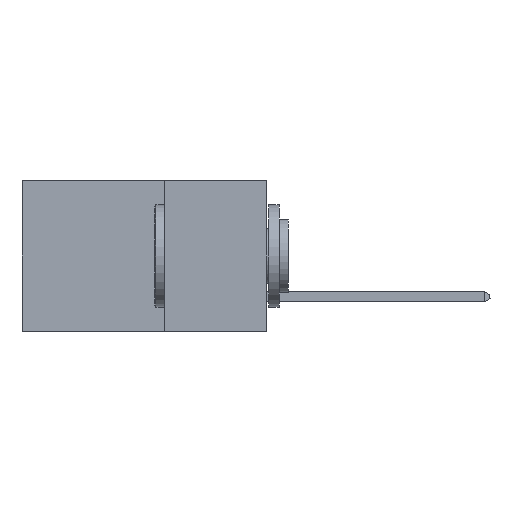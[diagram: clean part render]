
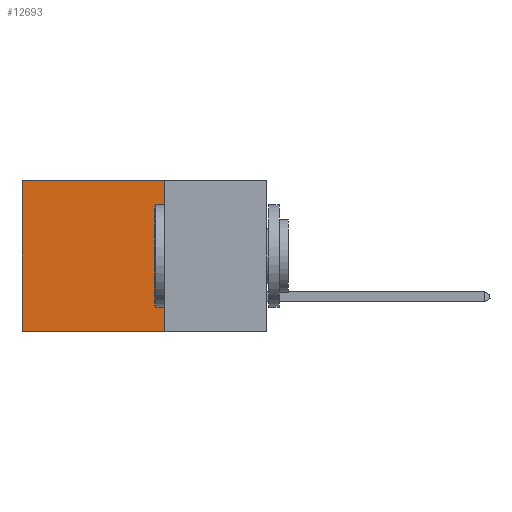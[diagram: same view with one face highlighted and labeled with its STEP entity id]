
A CAD part, left-side view. The second image highlights one B-rep face of the part: STEP entity #12693.
In plain terms, the highlighted planar face has unit normal (-1, 0, 0).
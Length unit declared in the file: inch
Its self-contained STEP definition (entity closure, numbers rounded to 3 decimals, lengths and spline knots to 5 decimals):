
#248 = LINE ( 'NONE', #10820, #5855 ) ;
#444 = CARTESIAN_POINT ( 'NONE',  ( 0.2875, 0.6, 0. ) ) ;
#707 = CARTESIAN_POINT ( 'NONE',  ( 0.2875, 0.6, -0.37 ) ) ;
#848 = ORIENTED_EDGE ( 'NONE', *, *, #1174, .T. ) ;
#1150 = EDGE_CURVE ( 'NONE', #14687, #1339, #15746, .T. ) ;
#1174 = EDGE_CURVE ( 'NONE', #4764, #14687, #248, .T. ) ;
#1325 = LINE ( 'NONE', #12075, #5479 ) ;
#1339 = VERTEX_POINT ( 'NONE', #707 ) ;
#1857 = CARTESIAN_POINT ( 'NONE',  ( 0.2875, 0.25, 0. ) ) ;
#2136 = LINE ( 'NONE', #1857, #9695 ) ;
#2764 = VERTEX_POINT ( 'NONE', #3407 ) ;
#3035 = CARTESIAN_POINT ( 'NONE',  ( 0.2875, 0.6, 0. ) ) ;
#3171 = DIRECTION ( 'NONE',  ( 0., 1., 0. ) ) ;
#3407 = CARTESIAN_POINT ( 'NONE',  ( 0.2875, 0.25, -0.37 ) ) ;
#4142 = EDGE_CURVE ( 'NONE', #4764, #2764, #2136, .T. ) ;
#4764 = VERTEX_POINT ( 'NONE', #6896 ) ;
#5479 = VECTOR ( 'NONE', #3171, 39.37008 ) ;
#5855 = VECTOR ( 'NONE', #9443, 39.37008 ) ;
#6426 = CARTESIAN_POINT ( 'NONE',  ( 0.2875, 0.25, 0. ) ) ;
#6896 = CARTESIAN_POINT ( 'NONE',  ( 0.2875, 0.25, 0. ) ) ;
#7521 = EDGE_LOOP ( 'NONE', ( #8079, #8293, #14871, #848 ) ) ;
#7677 = DIRECTION ( 'NONE',  ( 0., 0., -1. ) ) ;
#8079 = ORIENTED_EDGE ( 'NONE', *, *, #1150, .T. ) ;
#8144 = FACE_OUTER_BOUND ( 'NONE', #7521, .T. ) ;
#8293 = ORIENTED_EDGE ( 'NONE', *, *, #14139, .F. ) ;
#9443 = DIRECTION ( 'NONE',  ( 0., 1., 0. ) ) ;
#9467 = DIRECTION ( 'NONE',  ( 0., 0., -1. ) ) ;
#9695 = VECTOR ( 'NONE', #9467, 39.37008 ) ;
#10820 = CARTESIAN_POINT ( 'NONE',  ( 0.2875, 0.25, 0. ) ) ;
#11188 = AXIS2_PLACEMENT_3D ( 'NONE', #6426, #15168, #7677 ) ;
#11527 = PLANE ( 'NONE',  #11188 ) ;
#12075 = CARTESIAN_POINT ( 'NONE',  ( 0.2875, 0.25, -0.37 ) ) ;
#12596 = VECTOR ( 'NONE', #15952, 39.37008 ) ;
#12693 = ADVANCED_FACE ( 'NONE', ( #8144 ), #11527, .F. ) ;
#14139 = EDGE_CURVE ( 'NONE', #2764, #1339, #1325, .T. ) ;
#14687 = VERTEX_POINT ( 'NONE', #3035 ) ;
#14871 = ORIENTED_EDGE ( 'NONE', *, *, #4142, .F. ) ;
#15168 = DIRECTION ( 'NONE',  ( 1., 0., 0. ) ) ;
#15746 = LINE ( 'NONE', #444, #12596 ) ;
#15952 = DIRECTION ( 'NONE',  ( 0., 0., -1. ) ) ;
